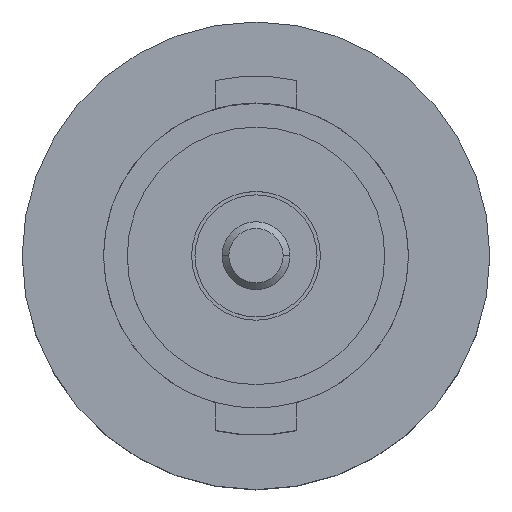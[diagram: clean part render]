
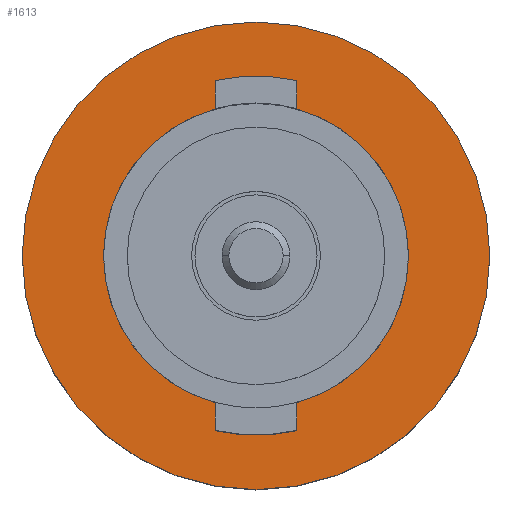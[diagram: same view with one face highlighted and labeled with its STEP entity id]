
A CAD part, top view. The second image highlights one B-rep face of the part: STEP entity #1613.
In plain terms, the highlighted planar face has unit normal (0, 0, 1).
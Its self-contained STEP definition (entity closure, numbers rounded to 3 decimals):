
#8 = LINE ( 'NONE', #663, #1247 ) ;
#17 = LINE ( 'NONE', #673, #485 ) ;
#21 = VERTEX_POINT ( 'NONE', #216 ) ;
#29 = ORIENTED_EDGE ( 'NONE', *, *, #1925, .F. ) ;
#33 = DIRECTION ( 'NONE',  ( 0., 0., 1. ) ) ;
#95 = ORIENTED_EDGE ( 'NONE', *, *, #1213, .F. ) ;
#100 = ORIENTED_EDGE ( 'NONE', *, *, #510, .F. ) ;
#114 = CARTESIAN_POINT ( 'NONE',  ( 60., -60., 30. ) ) ;
#118 = DIRECTION ( 'NONE',  ( 1., 0., 0. ) ) ;
#121 = EDGE_CURVE ( 'NONE', #2085, #483, #1000, .T. ) ;
#137 = EDGE_LOOP ( 'NONE', ( #100, #95, #29, #1614, #1524, #2206, #2218, #1311, #1430, #246 ) ) ;
#190 = CARTESIAN_POINT ( 'NONE',  ( 60.6, -57.419, 30. ) ) ;
#216 = CARTESIAN_POINT ( 'NONE',  ( 59.4, -57.419, 30. ) ) ;
#246 = ORIENTED_EDGE ( 'NONE', *, *, #1166, .F. ) ;
#261 = LINE ( 'NONE', #950, #1009 ) ;
#265 = CARTESIAN_POINT ( 'NONE',  ( 60.6, -57.831, 30. ) ) ;
#271 = PLANE ( 'NONE',  #1444 ) ;
#272 = EDGE_CURVE ( 'NONE', #2097, #285, #1222, .T. ) ;
#285 = VERTEX_POINT ( 'NONE', #878 ) ;
#310 = CARTESIAN_POINT ( 'NONE',  ( 56.55, -60., 30. ) ) ;
#341 = VECTOR ( 'NONE', #2106, 1000. ) ;
#375 = CARTESIAN_POINT ( 'NONE',  ( 60., -60., 30. ) ) ;
#403 = VERTEX_POINT ( 'NONE', #310 ) ;
#405 = ORIENTED_EDGE ( 'NONE', *, *, #450, .F. ) ;
#414 = VERTEX_POINT ( 'NONE', #1003 ) ;
#424 = CIRCLE ( 'NONE', #1640, 3.45 ) ;
#429 = DIRECTION ( 'NONE',  ( -0.226, -0.974, 0. ) ) ;
#433 = CARTESIAN_POINT ( 'NONE',  ( 60., -60., 30. ) ) ;
#450 = EDGE_CURVE ( 'NONE', #916, #403, #1792, .T. ) ;
#483 = VERTEX_POINT ( 'NONE', #1204 ) ;
#485 = VECTOR ( 'NONE', #1375, 1000. ) ;
#506 = DIRECTION ( 'NONE',  ( 1., 0., 0. ) ) ;
#509 = CARTESIAN_POINT ( 'NONE',  ( 60., -60., 30. ) ) ;
#510 = EDGE_CURVE ( 'NONE', #776, #21, #1748, .T. ) ;
#663 = CARTESIAN_POINT ( 'NONE',  ( 59.4, -62.169, 30. ) ) ;
#673 = CARTESIAN_POINT ( 'NONE',  ( 59.4, -57.419, 30. ) ) ;
#684 = LINE ( 'NONE', #1388, #341 ) ;
#691 = DIRECTION ( 'NONE',  ( -0.267, 0.964, 0. ) ) ;
#692 = CARTESIAN_POINT ( 'NONE',  ( 60., -60., 30. ) ) ;
#734 = CARTESIAN_POINT ( 'NONE',  ( 59.4, -62.169, 30. ) ) ;
#736 = EDGE_CURVE ( 'NONE', #414, #1467, #1496, .T. ) ;
#776 = VERTEX_POINT ( 'NONE', #190 ) ;
#782 = DIRECTION ( 'NONE',  ( 0., 0., 1. ) ) ;
#787 = CIRCLE ( 'NONE', #809, 2.25 ) ;
#809 = AXIS2_PLACEMENT_3D ( 'NONE', #114, #782, #1497 ) ;
#878 = CARTESIAN_POINT ( 'NONE',  ( 57.75, -60., 30. ) ) ;
#916 = VERTEX_POINT ( 'NONE', #2157 ) ;
#950 = CARTESIAN_POINT ( 'NONE',  ( 60.6, -62.581, 30. ) ) ;
#960 = CARTESIAN_POINT ( 'NONE',  ( 60., -60., 30. ) ) ;
#998 = EDGE_CURVE ( 'NONE', #285, #1230, #787, .T. ) ;
#1000 = CIRCLE ( 'NONE', #1002, 2.65 ) ;
#1002 = AXIS2_PLACEMENT_3D ( 'NONE', #1291, #2007, #429 ) ;
#1003 = CARTESIAN_POINT ( 'NONE',  ( 60.6, -62.169, 30. ) ) ;
#1009 = VECTOR ( 'NONE', #1664, 1000. ) ;
#1068 = DIRECTION ( 'NONE',  ( 0., 0., 1. ) ) ;
#1118 = DIRECTION ( 'NONE',  ( 0., 0., -1. ) ) ;
#1128 = FACE_OUTER_BOUND ( 'NONE', #1749, .T. ) ;
#1166 = EDGE_CURVE ( 'NONE', #21, #2097, #17, .T. ) ;
#1196 = DIRECTION ( 'NONE',  ( 0., 0., 1. ) ) ;
#1201 = ORIENTED_EDGE ( 'NONE', *, *, #1578, .F. ) ;
#1204 = CARTESIAN_POINT ( 'NONE',  ( 60.6, -62.581, 30. ) ) ;
#1213 = EDGE_CURVE ( 'NONE', #1579, #776, #684, .T. ) ;
#1222 = CIRCLE ( 'NONE', #1223, 2.25 ) ;
#1223 = AXIS2_PLACEMENT_3D ( 'NONE', #1580, #33, #691 ) ;
#1230 = VERTEX_POINT ( 'NONE', #734 ) ;
#1247 = VECTOR ( 'NONE', #1368, 1000. ) ;
#1291 = CARTESIAN_POINT ( 'NONE',  ( 60., -60., 30. ) ) ;
#1311 = ORIENTED_EDGE ( 'NONE', *, *, #998, .F. ) ;
#1368 = DIRECTION ( 'NONE',  ( 0., -1., 0. ) ) ;
#1372 = CARTESIAN_POINT ( 'NONE',  ( 60., -60., 30. ) ) ;
#1375 = DIRECTION ( 'NONE',  ( 0., -1., 0. ) ) ;
#1388 = CARTESIAN_POINT ( 'NONE',  ( 60.6, -57.831, 30. ) ) ;
#1397 = DIRECTION ( 'NONE',  ( 0., 0., 1. ) ) ;
#1430 = ORIENTED_EDGE ( 'NONE', *, *, #272, .F. ) ;
#1444 = AXIS2_PLACEMENT_3D ( 'NONE', #960, #1675, #118 ) ;
#1467 = VERTEX_POINT ( 'NONE', #2117 ) ;
#1496 = CIRCLE ( 'NONE', #1520, 2.25 ) ;
#1497 = DIRECTION ( 'NONE',  ( -1., 0., 0. ) ) ;
#1520 = AXIS2_PLACEMENT_3D ( 'NONE', #509, #1196, #1915 ) ;
#1524 = ORIENTED_EDGE ( 'NONE', *, *, #2056, .F. ) ;
#1578 = EDGE_CURVE ( 'NONE', #403, #916, #424, .T. ) ;
#1579 = VERTEX_POINT ( 'NONE', #265 ) ;
#1580 = CARTESIAN_POINT ( 'NONE',  ( 60., -60., 30. ) ) ;
#1613 = ADVANCED_FACE ( 'NONE', ( #1128, #1848 ), #271, .T. ) ;
#1614 = ORIENTED_EDGE ( 'NONE', *, *, #736, .F. ) ;
#1640 = AXIS2_PLACEMENT_3D ( 'NONE', #433, #1118, #1840 ) ;
#1664 = DIRECTION ( 'NONE',  ( 0., 1., 0. ) ) ;
#1675 = DIRECTION ( 'NONE',  ( 0., 0., 1. ) ) ;
#1721 = AXIS2_PLACEMENT_3D ( 'NONE', #375, #1068, #1788 ) ;
#1748 = CIRCLE ( 'NONE', #1750, 2.65 ) ;
#1749 = EDGE_LOOP ( 'NONE', ( #1201, #405 ) ) ;
#1750 = AXIS2_PLACEMENT_3D ( 'NONE', #692, #1397, #2115 ) ;
#1760 = EDGE_CURVE ( 'NONE', #1230, #2085, #8, .T. ) ;
#1788 = DIRECTION ( 'NONE',  ( 1., 0., 0. ) ) ;
#1792 = CIRCLE ( 'NONE', #1794, 3.45 ) ;
#1794 = AXIS2_PLACEMENT_3D ( 'NONE', #1372, #2088, #506 ) ;
#1840 = DIRECTION ( 'NONE',  ( -1., 0., 0. ) ) ;
#1845 = CARTESIAN_POINT ( 'NONE',  ( 59.4, -62.581, 30. ) ) ;
#1848 = FACE_BOUND ( 'NONE', #137, .T. ) ;
#1915 = DIRECTION ( 'NONE',  ( 0.267, -0.964, 0. ) ) ;
#1925 = EDGE_CURVE ( 'NONE', #1467, #1579, #2239, .T. ) ;
#2007 = DIRECTION ( 'NONE',  ( 0., 0., 1. ) ) ;
#2056 = EDGE_CURVE ( 'NONE', #483, #414, #261, .T. ) ;
#2085 = VERTEX_POINT ( 'NONE', #1845 ) ;
#2088 = DIRECTION ( 'NONE',  ( 0., 0., -1. ) ) ;
#2097 = VERTEX_POINT ( 'NONE', #2210 ) ;
#2106 = DIRECTION ( 'NONE',  ( 0., 1., 0. ) ) ;
#2115 = DIRECTION ( 'NONE',  ( 0., 1., 0. ) ) ;
#2117 = CARTESIAN_POINT ( 'NONE',  ( 62.25, -60., 30. ) ) ;
#2157 = CARTESIAN_POINT ( 'NONE',  ( 63.45, -60., 30. ) ) ;
#2206 = ORIENTED_EDGE ( 'NONE', *, *, #121, .F. ) ;
#2210 = CARTESIAN_POINT ( 'NONE',  ( 59.4, -57.831, 30. ) ) ;
#2218 = ORIENTED_EDGE ( 'NONE', *, *, #1760, .F. ) ;
#2239 = CIRCLE ( 'NONE', #1721, 2.25 ) ;
